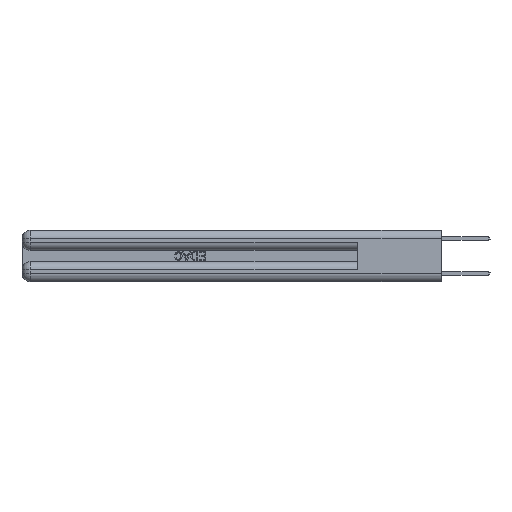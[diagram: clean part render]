
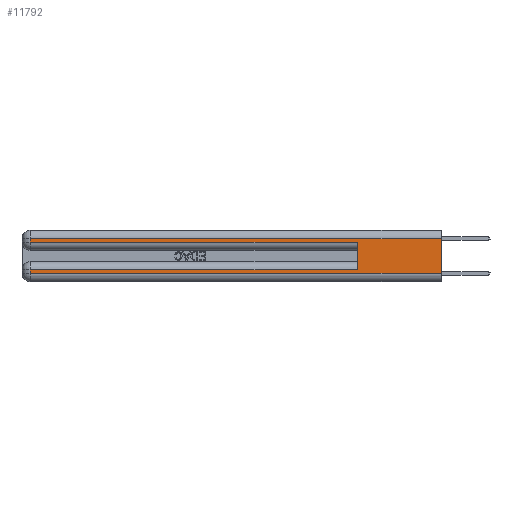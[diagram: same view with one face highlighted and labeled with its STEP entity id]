
A CAD part, left-side view. The second image highlights one B-rep face of the part: STEP entity #11792.
In plain terms, the highlighted planar face has unit normal (-1, 0, 0).
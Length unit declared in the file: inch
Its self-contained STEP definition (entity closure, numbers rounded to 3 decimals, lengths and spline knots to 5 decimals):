
#348 = CARTESIAN_POINT ( 'NONE',  ( 0., 2.94, 0.37 ) ) ;
#631 = ORIENTED_EDGE ( 'NONE', *, *, #4551, .T. ) ;
#1410 = VERTEX_POINT ( 'NONE', #8028 ) ;
#2255 = EDGE_CURVE ( 'NONE', #26228, #11036, #7816, .T. ) ;
#2757 = CARTESIAN_POINT ( 'NONE',  ( 0., 2.94, 0.37 ) ) ;
#3187 = DIRECTION ( 'NONE',  ( 0., 1., 0. ) ) ;
#3471 = CARTESIAN_POINT ( 'NONE',  ( 0., 0., 0.31 ) ) ;
#4098 = LINE ( 'NONE', #16358, #27099 ) ;
#4500 = DIRECTION ( 'NONE',  ( 1., 0., 0. ) ) ;
#4551 = EDGE_CURVE ( 'NONE', #11036, #27535, #15279, .T. ) ;
#4627 = CARTESIAN_POINT ( 'NONE',  ( 0., 0., 0.37 ) ) ;
#4734 = LINE ( 'NONE', #2757, #7083 ) ;
#5616 = VECTOR ( 'NONE', #17058, 39.37008 ) ;
#5636 = VERTEX_POINT ( 'NONE', #9385 ) ;
#6613 = DIRECTION ( 'NONE',  ( 0., 0., -1. ) ) ;
#6631 = AXIS2_PLACEMENT_3D ( 'NONE', #4627, #4500, #6613 ) ;
#7024 = FACE_OUTER_BOUND ( 'NONE', #20897, .T. ) ;
#7083 = VECTOR ( 'NONE', #17302, 39.37008 ) ;
#7204 = ORIENTED_EDGE ( 'NONE', *, *, #12909, .F. ) ;
#7816 = LINE ( 'NONE', #3471, #22316 ) ;
#7824 = CARTESIAN_POINT ( 'NONE',  ( 0., 2.94, 0.285 ) ) ;
#8028 = CARTESIAN_POINT ( 'NONE',  ( 0., 0.6, 0.285 ) ) ;
#8913 = VECTOR ( 'NONE', #24984, 39.37008 ) ;
#9030 = EDGE_CURVE ( 'NONE', #24255, #5636, #14533, .T. ) ;
#9385 = CARTESIAN_POINT ( 'NONE',  ( 0., 2.94, 0.085 ) ) ;
#10528 = ORIENTED_EDGE ( 'NONE', *, *, #12274, .T. ) ;
#11036 = VERTEX_POINT ( 'NONE', #18302 ) ;
#11792 = ADVANCED_FACE ( 'NONE', ( #7024 ), #19582, .F. ) ;
#12265 = DIRECTION ( 'NONE',  ( 0., 0., 1. ) ) ;
#12274 = EDGE_CURVE ( 'NONE', #5636, #19285, #4734, .T. ) ;
#12764 = ORIENTED_EDGE ( 'NONE', *, *, #22096, .T. ) ;
#12909 = EDGE_CURVE ( 'NONE', #26228, #18270, #20612, .T. ) ;
#14533 = LINE ( 'NONE', #23156, #18293 ) ;
#15279 = LINE ( 'NONE', #348, #22043 ) ;
#15547 = VECTOR ( 'NONE', #16245, 39.37008 ) ;
#16245 = DIRECTION ( 'NONE',  ( 0., -1., 0. ) ) ;
#16358 = CARTESIAN_POINT ( 'NONE',  ( 0., 0.6, 0.145 ) ) ;
#16530 = LINE ( 'NONE', #25297, #15547 ) ;
#16911 = CARTESIAN_POINT ( 'NONE',  ( 0., 0.6, 0.085 ) ) ;
#17058 = DIRECTION ( 'NONE',  ( 0., -1., 0. ) ) ;
#17302 = DIRECTION ( 'NONE',  ( 0., 0., -1. ) ) ;
#17393 = CARTESIAN_POINT ( 'NONE',  ( 0., 0., 0.06 ) ) ;
#18270 = VERTEX_POINT ( 'NONE', #17393 ) ;
#18293 = VECTOR ( 'NONE', #21041, 39.37008 ) ;
#18302 = CARTESIAN_POINT ( 'NONE',  ( 0., 2.94, 0.31 ) ) ;
#18303 = ORIENTED_EDGE ( 'NONE', *, *, #23565, .T. ) ;
#19285 = VERTEX_POINT ( 'NONE', #24164 ) ;
#19582 = PLANE ( 'NONE',  #6631 ) ;
#20612 = LINE ( 'NONE', #27115, #8913 ) ;
#20835 = ORIENTED_EDGE ( 'NONE', *, *, #9030, .T. ) ;
#20897 = EDGE_LOOP ( 'NONE', ( #7204, #23030, #631, #18303, #23617, #20835, #10528, #12764 ) ) ;
#21041 = DIRECTION ( 'NONE',  ( 0., 1., 0. ) ) ;
#21294 = CARTESIAN_POINT ( 'NONE',  ( 0., 0., 0.06 ) ) ;
#22043 = VECTOR ( 'NONE', #23618, 39.37008 ) ;
#22096 = EDGE_CURVE ( 'NONE', #19285, #18270, #23421, .T. ) ;
#22316 = VECTOR ( 'NONE', #3187, 39.37008 ) ;
#23030 = ORIENTED_EDGE ( 'NONE', *, *, #2255, .T. ) ;
#23156 = CARTESIAN_POINT ( 'NONE',  ( 0., 0., 0.085 ) ) ;
#23421 = LINE ( 'NONE', #21294, #5616 ) ;
#23565 = EDGE_CURVE ( 'NONE', #27535, #1410, #16530, .T. ) ;
#23617 = ORIENTED_EDGE ( 'NONE', *, *, #27309, .F. ) ;
#23618 = DIRECTION ( 'NONE',  ( 0., 0., -1. ) ) ;
#24164 = CARTESIAN_POINT ( 'NONE',  ( 0., 2.94, 0.06 ) ) ;
#24255 = VERTEX_POINT ( 'NONE', #16911 ) ;
#24984 = DIRECTION ( 'NONE',  ( 0., 0., -1. ) ) ;
#25297 = CARTESIAN_POINT ( 'NONE',  ( 0., 0., 0.285 ) ) ;
#25937 = CARTESIAN_POINT ( 'NONE',  ( 0., 0., 0.31 ) ) ;
#26228 = VERTEX_POINT ( 'NONE', #25937 ) ;
#27099 = VECTOR ( 'NONE', #12265, 39.37008 ) ;
#27115 = CARTESIAN_POINT ( 'NONE',  ( 0., 0., 0.37 ) ) ;
#27309 = EDGE_CURVE ( 'NONE', #24255, #1410, #4098, .T. ) ;
#27535 = VERTEX_POINT ( 'NONE', #7824 ) ;
